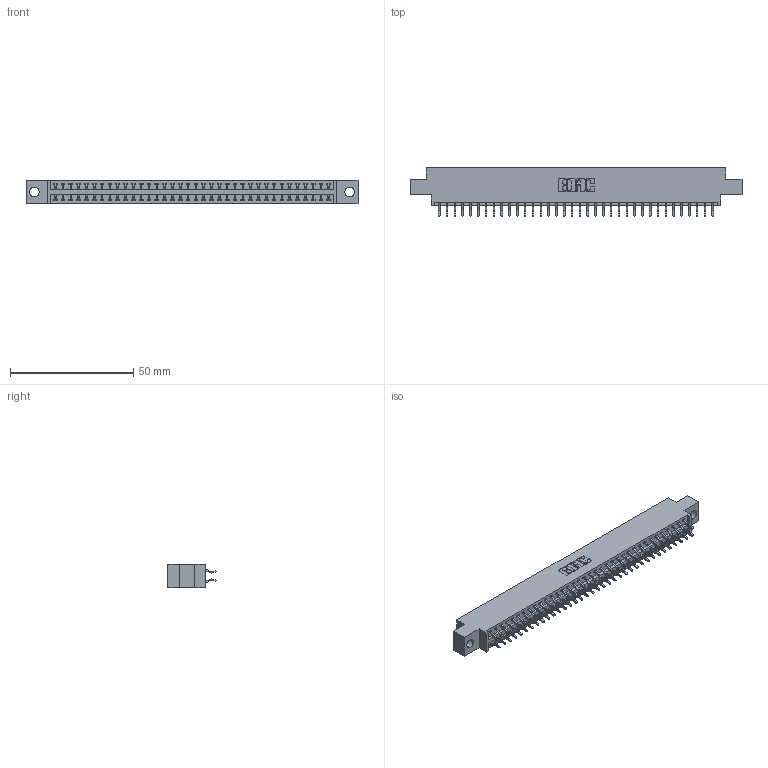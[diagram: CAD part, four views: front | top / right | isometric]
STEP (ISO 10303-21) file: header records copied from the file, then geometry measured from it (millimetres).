
FILE_DESCRIPTION (( 'STEP AP203' ), '1' );
FILE_NAME ('346-072-556-804.STEP', '2022-05-25T00:38:41', ( '' ), ( '' ), 'SwSTEP 2.0', 'SolidWorks 2020', '' );
FILE_SCHEMA (( 'CONFIG_CONTROL_DESIGN' ));
Length unit declared in the file: inch
Products named in the file (3): 345-292-001_556 Tail; 346 Part_0.170 Offset - 0.156 Dia-TH; 346-072-556-804
Assembly tree (73 placements, depth 2):
  346-072-556-804
    346 Part_0.170 Offset - 0.156 Dia-TH
    345-292-001_556 Tail  x72
Bounding box: 134.87 x 19.57 x 9.4 mm (x, y, z)
Volume: 12841.9 mm3; surface area: 17518.3 mm2
Topology: 73 solids, 73 shells, 4316 faces, 12833 edges, 8458 vertices
Faces by surface type: plane 2902, cylinder 1414
Entity records: 25073 total; most frequent: CARTESIAN_POINT 4162, ORIENTED_EDGE 4082, DIRECTION 3705, EDGE_CURVE 2041, LINE 1757, VECTOR 1757, VERTEX_POINT 1358, AXIS2_PLACEMENT_3D 974
